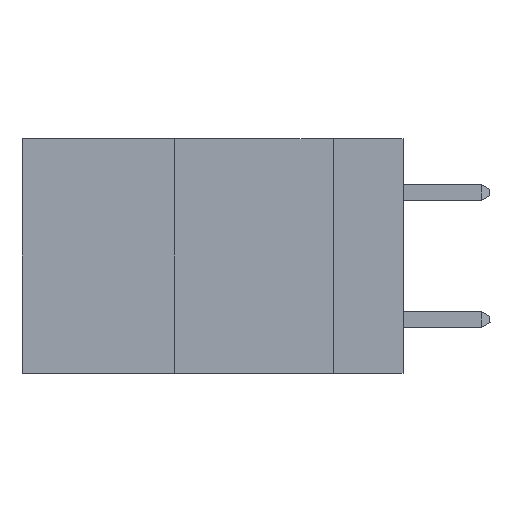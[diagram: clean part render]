
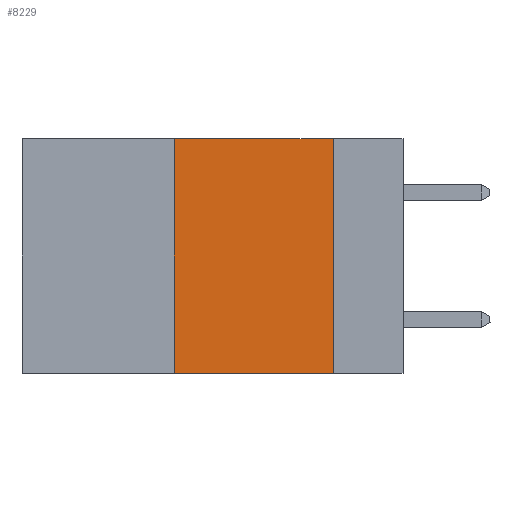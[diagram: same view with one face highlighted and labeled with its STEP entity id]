
A CAD part, left-side view. The second image highlights one B-rep face of the part: STEP entity #8229.
In plain terms, the highlighted planar face has unit normal (-1, 0, 0).
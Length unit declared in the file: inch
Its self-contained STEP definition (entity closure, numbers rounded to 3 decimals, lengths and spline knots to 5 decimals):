
#731 = ORIENTED_EDGE ( 'NONE', *, *, #12079, .T. ) ;
#979 = LINE ( 'NONE', #11276, #5661 ) ;
#1587 = CARTESIAN_POINT ( 'NONE',  ( 0., 0.11, -0.37 ) ) ;
#2231 = LINE ( 'NONE', #3598, #9017 ) ;
#2314 = EDGE_CURVE ( 'NONE', #13093, #6007, #8668, .T. ) ;
#2324 = DIRECTION ( 'NONE',  ( 0., -1., 0. ) ) ;
#2537 = DIRECTION ( 'NONE',  ( 0., 0., -1. ) ) ;
#3216 = DIRECTION ( 'NONE',  ( 0., -1., 0. ) ) ;
#3263 = VECTOR ( 'NONE', #11148, 39.37008 ) ;
#3598 = CARTESIAN_POINT ( 'NONE',  ( 0., 0.11, 0. ) ) ;
#3649 = PLANE ( 'NONE',  #9757 ) ;
#4730 = CARTESIAN_POINT ( 'NONE',  ( 0., 0.36, 0. ) ) ;
#5661 = VECTOR ( 'NONE', #2324, 39.37008 ) ;
#5901 = VERTEX_POINT ( 'NONE', #1587 ) ;
#6007 = VERTEX_POINT ( 'NONE', #8307 ) ;
#7597 = CARTESIAN_POINT ( 'NONE',  ( 0., 0.11, 0. ) ) ;
#7667 = ORIENTED_EDGE ( 'NONE', *, *, #8771, .F. ) ;
#8229 = ADVANCED_FACE ( 'NONE', ( #8344 ), #3649, .F. ) ;
#8307 = CARTESIAN_POINT ( 'NONE',  ( 0., 0.36, 0. ) ) ;
#8344 = FACE_OUTER_BOUND ( 'NONE', #10072, .T. ) ;
#8659 = ORIENTED_EDGE ( 'NONE', *, *, #10471, .F. ) ;
#8668 = LINE ( 'NONE', #4730, #3263 ) ;
#8771 = EDGE_CURVE ( 'NONE', #9890, #5901, #2231, .T. ) ;
#9017 = VECTOR ( 'NONE', #13437, 39.37008 ) ;
#9121 = CARTESIAN_POINT ( 'NONE',  ( 0., 0.36, -0.37 ) ) ;
#9162 = ORIENTED_EDGE ( 'NONE', *, *, #2314, .F. ) ;
#9455 = LINE ( 'NONE', #11040, #11874 ) ;
#9757 = AXIS2_PLACEMENT_3D ( 'NONE', #10462, #10419, #2537 ) ;
#9890 = VERTEX_POINT ( 'NONE', #7597 ) ;
#10072 = EDGE_LOOP ( 'NONE', ( #7667, #8659, #9162, #731 ) ) ;
#10419 = DIRECTION ( 'NONE',  ( 1., 0., 0. ) ) ;
#10462 = CARTESIAN_POINT ( 'NONE',  ( 0., 0.6, 0. ) ) ;
#10471 = EDGE_CURVE ( 'NONE', #6007, #9890, #9455, .T. ) ;
#11040 = CARTESIAN_POINT ( 'NONE',  ( 0., 0.6, 0. ) ) ;
#11148 = DIRECTION ( 'NONE',  ( 0., 0., 1. ) ) ;
#11276 = CARTESIAN_POINT ( 'NONE',  ( 0., 0.6, -0.37 ) ) ;
#11874 = VECTOR ( 'NONE', #3216, 39.37008 ) ;
#12079 = EDGE_CURVE ( 'NONE', #13093, #5901, #979, .T. ) ;
#13093 = VERTEX_POINT ( 'NONE', #9121 ) ;
#13437 = DIRECTION ( 'NONE',  ( 0., 0., -1. ) ) ;
